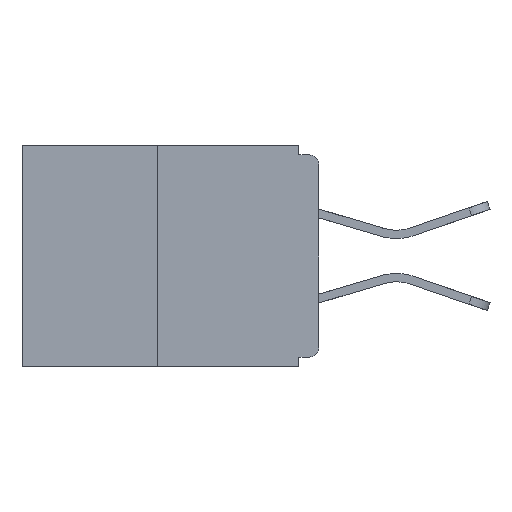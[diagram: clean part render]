
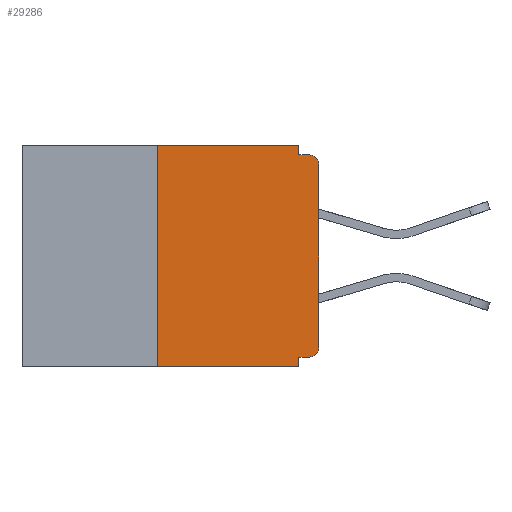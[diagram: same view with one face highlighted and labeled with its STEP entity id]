
A CAD part, left-side view. The second image highlights one B-rep face of the part: STEP entity #29286.
In plain terms, the highlighted planar face has unit normal (-1, 0, 0).
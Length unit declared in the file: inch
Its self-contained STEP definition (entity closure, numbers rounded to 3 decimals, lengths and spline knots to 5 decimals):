
#77 = DIRECTION ( 'NONE',  ( -1., 0., 0. ) ) ;
#190 = AXIS2_PLACEMENT_3D ( 'NONE', #219, #19968, #24915 ) ;
#219 = CARTESIAN_POINT ( 'NONE',  ( 0., 0.015, -0.313 ) ) ;
#976 = EDGE_CURVE ( 'NONE', #24024, #9142, #14070, .T. ) ;
#1319 = VERTEX_POINT ( 'NONE', #9756 ) ;
#1359 = CARTESIAN_POINT ( 'NONE',  ( 0., 0.031, -0.343 ) ) ;
#1373 = VECTOR ( 'NONE', #28018, 39.37008 ) ;
#2134 = LINE ( 'NONE', #8452, #7943 ) ;
#2459 = DIRECTION ( 'NONE',  ( 0., 0., -1. ) ) ;
#3140 = VECTOR ( 'NONE', #27273, 39.37008 ) ;
#3155 = DIRECTION ( 'NONE',  ( 0., -1., 0. ) ) ;
#3624 = CARTESIAN_POINT ( 'NONE',  ( 0., 0.031, -0.328 ) ) ;
#3813 = VECTOR ( 'NONE', #24738, 39.37008 ) ;
#3821 = AXIS2_PLACEMENT_3D ( 'NONE', #14025, #77, #2459 ) ;
#5082 = EDGE_CURVE ( 'NONE', #31522, #9142, #13846, .T. ) ;
#6177 = PLANE ( 'NONE',  #12704 ) ;
#7493 = CARTESIAN_POINT ( 'NONE',  ( 0., 0., -0.328 ) ) ;
#7532 = VERTEX_POINT ( 'NONE', #23295 ) ;
#7943 = VECTOR ( 'NONE', #18879, 39.37008 ) ;
#8184 = VERTEX_POINT ( 'NONE', #18932 ) ;
#8452 = CARTESIAN_POINT ( 'NONE',  ( 0., 0., 0. ) ) ;
#8763 = ORIENTED_EDGE ( 'NONE', *, *, #19868, .F. ) ;
#8835 = ORIENTED_EDGE ( 'NONE', *, *, #13870, .T. ) ;
#8931 = DIRECTION ( 'NONE',  ( 0., 0., 1. ) ) ;
#9142 = VERTEX_POINT ( 'NONE', #1359 ) ;
#9322 = ORIENTED_EDGE ( 'NONE', *, *, #25575, .T. ) ;
#9756 = CARTESIAN_POINT ( 'NONE',  ( 0., 0.015, -0.328 ) ) ;
#9762 = EDGE_CURVE ( 'NONE', #31522, #7532, #25866, .T. ) ;
#9801 = FACE_OUTER_BOUND ( 'NONE', #24073, .T. ) ;
#9859 = VERTEX_POINT ( 'NONE', #23812 ) ;
#10071 = VECTOR ( 'NONE', #8931, 39.37008 ) ;
#11873 = ORIENTED_EDGE ( 'NONE', *, *, #976, .F. ) ;
#11907 = LINE ( 'NONE', #29119, #18100 ) ;
#12704 = AXIS2_PLACEMENT_3D ( 'NONE', #18354, #28224, #15949 ) ;
#12795 = ORIENTED_EDGE ( 'NONE', *, *, #9762, .F. ) ;
#13452 = DIRECTION ( 'NONE',  ( 0., -1., 0. ) ) ;
#13734 = CIRCLE ( 'NONE', #190, 0.015 ) ;
#13846 = LINE ( 'NONE', #17947, #18099 ) ;
#13870 = EDGE_CURVE ( 'NONE', #8184, #15560, #16966, .T. ) ;
#14025 = CARTESIAN_POINT ( 'NONE',  ( 0., 0.015, -0.03 ) ) ;
#14054 = EDGE_CURVE ( 'NONE', #1319, #24024, #21928, .T. ) ;
#14070 = LINE ( 'NONE', #15635, #1373 ) ;
#15560 = VERTEX_POINT ( 'NONE', #23045 ) ;
#15635 = CARTESIAN_POINT ( 'NONE',  ( 0., 0.031, -0.343 ) ) ;
#15826 = CARTESIAN_POINT ( 'NONE',  ( 0., 0.25, 0. ) ) ;
#15949 = DIRECTION ( 'NONE',  ( 0., 0., -1. ) ) ;
#16966 = CIRCLE ( 'NONE', #3821, 0.015 ) ;
#17947 = CARTESIAN_POINT ( 'NONE',  ( 0., 0.46, -0.343 ) ) ;
#18099 = VECTOR ( 'NONE', #3155, 39.37008 ) ;
#18100 = VECTOR ( 'NONE', #21686, 39.37008 ) ;
#18192 = VERTEX_POINT ( 'NONE', #19609 ) ;
#18354 = CARTESIAN_POINT ( 'NONE',  ( 0., 0.46, 0. ) ) ;
#18716 = ORIENTED_EDGE ( 'NONE', *, *, #5082, .T. ) ;
#18879 = DIRECTION ( 'NONE',  ( 0., 0., 1. ) ) ;
#18932 = CARTESIAN_POINT ( 'NONE',  ( 0., 0., -0.03 ) ) ;
#19242 = EDGE_CURVE ( 'NONE', #27544, #8184, #2134, .T. ) ;
#19609 = CARTESIAN_POINT ( 'NONE',  ( 0., 0.031, 0. ) ) ;
#19868 = EDGE_CURVE ( 'NONE', #9859, #15560, #25277, .T. ) ;
#19967 = ORIENTED_EDGE ( 'NONE', *, *, #19242, .T. ) ;
#19968 = DIRECTION ( 'NONE',  ( -1., 0., 0. ) ) ;
#21686 = DIRECTION ( 'NONE',  ( 0., -1., 0. ) ) ;
#21928 = LINE ( 'NONE', #7493, #3813 ) ;
#22176 = VECTOR ( 'NONE', #13452, 39.37008 ) ;
#22268 = ORIENTED_EDGE ( 'NONE', *, *, #30598, .F. ) ;
#23045 = CARTESIAN_POINT ( 'NONE',  ( 0., 0.015, -0.015 ) ) ;
#23295 = CARTESIAN_POINT ( 'NONE',  ( 0., 0.25, 0. ) ) ;
#23343 = EDGE_CURVE ( 'NONE', #7532, #18192, #11907, .T. ) ;
#23812 = CARTESIAN_POINT ( 'NONE',  ( 0., 0.031, -0.015 ) ) ;
#24024 = VERTEX_POINT ( 'NONE', #3624 ) ;
#24073 = EDGE_LOOP ( 'NONE', ( #26224, #12795, #18716, #11873, #27349, #9322, #19967, #8835, #8763, #22268 ) ) ;
#24738 = DIRECTION ( 'NONE',  ( 0., 1., 0. ) ) ;
#24915 = DIRECTION ( 'NONE',  ( 0., 0., -1. ) ) ;
#25277 = LINE ( 'NONE', #28169, #22176 ) ;
#25344 = CARTESIAN_POINT ( 'NONE',  ( 0., 0., -0.313 ) ) ;
#25575 = EDGE_CURVE ( 'NONE', #1319, #27544, #13734, .T. ) ;
#25866 = LINE ( 'NONE', #15826, #10071 ) ;
#26224 = ORIENTED_EDGE ( 'NONE', *, *, #23343, .F. ) ;
#27047 = LINE ( 'NONE', #29615, #3140 ) ;
#27273 = DIRECTION ( 'NONE',  ( 0., 0., -1. ) ) ;
#27349 = ORIENTED_EDGE ( 'NONE', *, *, #14054, .F. ) ;
#27544 = VERTEX_POINT ( 'NONE', #25344 ) ;
#28018 = DIRECTION ( 'NONE',  ( 0., 0., -1. ) ) ;
#28169 = CARTESIAN_POINT ( 'NONE',  ( 0., 0., -0.015 ) ) ;
#28224 = DIRECTION ( 'NONE',  ( 1., 0., 0. ) ) ;
#29119 = CARTESIAN_POINT ( 'NONE',  ( 0., 0.46, 0. ) ) ;
#29286 = ADVANCED_FACE ( 'NONE', ( #9801 ), #6177, .F. ) ;
#29615 = CARTESIAN_POINT ( 'NONE',  ( 0., 0.031, 0. ) ) ;
#30598 = EDGE_CURVE ( 'NONE', #18192, #9859, #27047, .T. ) ;
#31501 = CARTESIAN_POINT ( 'NONE',  ( 0., 0.25, -0.343 ) ) ;
#31522 = VERTEX_POINT ( 'NONE', #31501 ) ;
